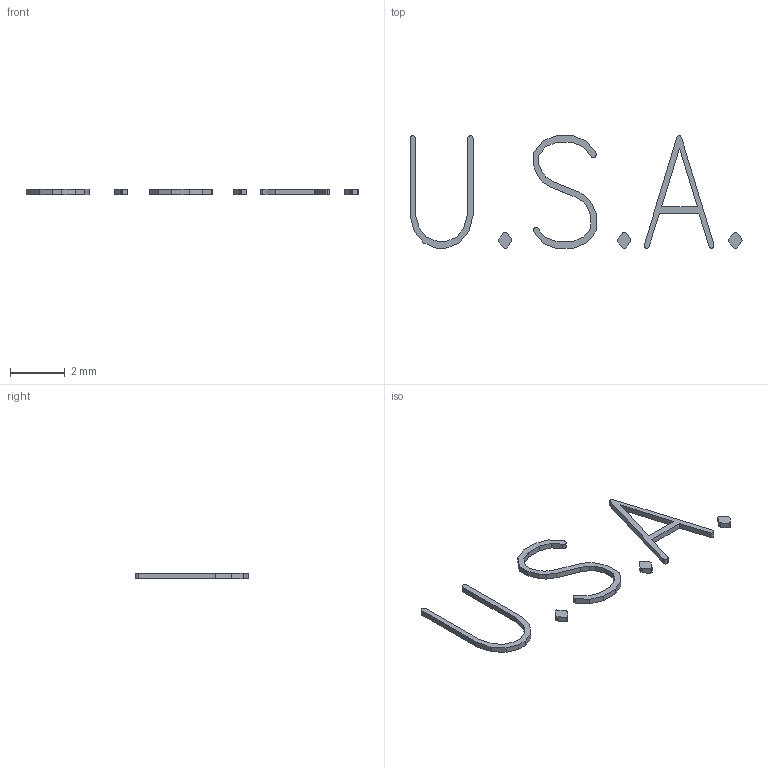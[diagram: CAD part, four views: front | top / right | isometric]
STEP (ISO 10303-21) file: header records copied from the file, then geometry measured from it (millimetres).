
FILE_DESCRIPTION (( 'STEP AP214' ), '1' );
FILE_NAME ('ENGRAVING FILL - USA.STEP', '2013-06-19T14:03:31', ( 'Asher' ), ( '' ), 'SwSTEP 2.0', 'SolidWorks 2013', '' );
FILE_SCHEMA (( 'AUTOMOTIVE_DESIGN' ));
Length unit declared in the file: millimetre
Products named in the file (1): ENGRAVING FILL - USA
Bounding box: 12.11 x 4.11 x 0.2 mm (x, y, z)
Volume: 1.3 mm3; surface area: 25 mm2
Topology: 6 solids, 6 shells, 136 faces, 372 edges, 248 vertices
Faces by surface type: plane 85, bspline 51
Entity records: 5057 total; most frequent: CARTESIAN_POINT 1872, ORIENTED_EDGE 744, DIRECTION 442, EDGE_CURVE 372, VECTOR 270, LINE 270, VERTEX_POINT 248, EDGE_LOOP 138
